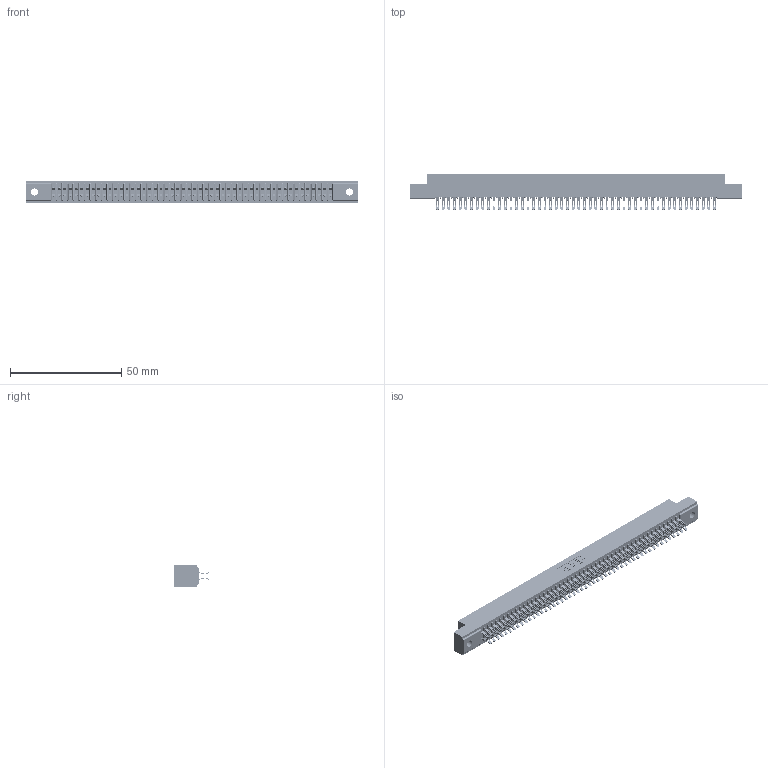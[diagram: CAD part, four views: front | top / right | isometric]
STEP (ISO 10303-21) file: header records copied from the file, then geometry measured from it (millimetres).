
FILE_DESCRIPTION (( 'STEP AP203' ), '1' );
FILE_NAME ('341-100-555-202.STEP', '2018-08-08T02:55:52', ( '' ), ( '' ), 'SwSTEP 2.0', 'SolidWorks 2016', '' );
FILE_SCHEMA (( 'CONFIG_CONTROL_DESIGN' ));
Length unit declared in the file: inch
Products named in the file (3): 341 Part_.128 (3.25) Dia Mounting Holes; 341-292-001_341-292-155; 341-100-555-202
Assembly tree (101 placements, depth 2):
  341-100-555-202
    341 Part_.128 (3.25) Dia Mounting Holes
    341-292-001_341-292-155  x100
Bounding box: 149.22 x 16.31 x 10.16 mm (x, y, z)
Volume: 11113.5 mm3; surface area: 20545.8 mm2
Topology: 101 solids, 101 shells, 7916 faces, 23666 edges, 15406 vertices
Faces by surface type: plane 4268, cylinder 3448, sphere 102, torus 98
Entity records: 59917 total; most frequent: CARTESIAN_POINT 9976, ORIENTED_EDGE 9904, DIRECTION 9666, EDGE_CURVE 4952, LINE 3994, VECTOR 3994, VERTEX_POINT 3130, AXIS2_PLACEMENT_3D 2836
